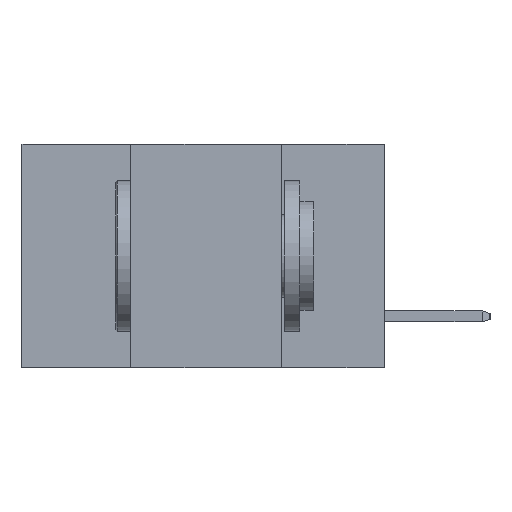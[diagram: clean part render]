
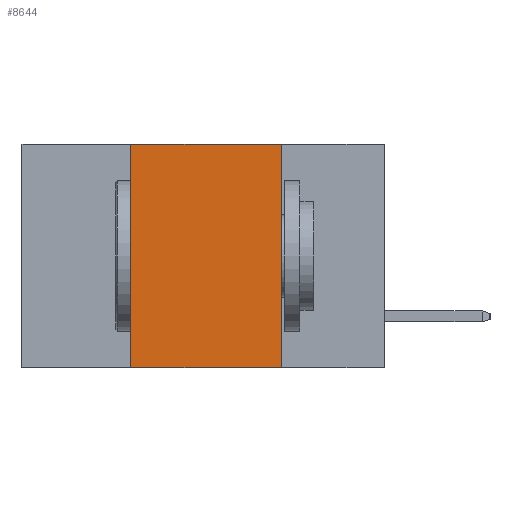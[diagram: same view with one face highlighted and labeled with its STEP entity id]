
A CAD part, left-side view. The second image highlights one B-rep face of the part: STEP entity #8644.
In plain terms, the highlighted planar face has unit normal (-1, 0, 0).
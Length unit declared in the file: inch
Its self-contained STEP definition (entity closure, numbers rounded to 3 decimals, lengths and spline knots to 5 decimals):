
#304 = LINE ( 'NONE', #5395, #17851 ) ;
#500 = DIRECTION ( 'NONE',  ( 1., 0., 0. ) ) ;
#922 = ORIENTED_EDGE ( 'NONE', *, *, #5301, .F. ) ;
#1385 = VECTOR ( 'NONE', #2786, 39.37008 ) ;
#1415 = ORIENTED_EDGE ( 'NONE', *, *, #14925, .F. ) ;
#1809 = CARTESIAN_POINT ( 'NONE',  ( 0., 0.17, 0. ) ) ;
#2786 = DIRECTION ( 'NONE',  ( 0., -1., 0. ) ) ;
#2829 = VECTOR ( 'NONE', #4533, 39.37008 ) ;
#3095 = CARTESIAN_POINT ( 'NONE',  ( 0., 0.6, -0.37 ) ) ;
#3645 = FACE_OUTER_BOUND ( 'NONE', #14759, .T. ) ;
#3710 = CARTESIAN_POINT ( 'NONE',  ( 0., 0.42, 0. ) ) ;
#3928 = CARTESIAN_POINT ( 'NONE',  ( 0., 0.42, -0.37 ) ) ;
#4533 = DIRECTION ( 'NONE',  ( 0., -1., 0. ) ) ;
#4705 = VECTOR ( 'NONE', #14823, 39.37008 ) ;
#5096 = AXIS2_PLACEMENT_3D ( 'NONE', #15878, #500, #10499 ) ;
#5301 = EDGE_CURVE ( 'NONE', #14714, #15538, #304, .T. ) ;
#5395 = CARTESIAN_POINT ( 'NONE',  ( 0., 0.17, 0. ) ) ;
#5481 = CARTESIAN_POINT ( 'NONE',  ( 0., 0.42, 0. ) ) ;
#5553 = DIRECTION ( 'NONE',  ( 0., 0., -1. ) ) ;
#8644 = ADVANCED_FACE ( 'NONE', ( #3645 ), #17155, .F. ) ;
#9843 = CARTESIAN_POINT ( 'NONE',  ( 0., 0.6, 0. ) ) ;
#10359 = LINE ( 'NONE', #3095, #2829 ) ;
#10499 = DIRECTION ( 'NONE',  ( 0., 0., -1. ) ) ;
#12109 = CARTESIAN_POINT ( 'NONE',  ( 0., 0.17, -0.37 ) ) ;
#12234 = EDGE_CURVE ( 'NONE', #13834, #15538, #10359, .T. ) ;
#12274 = ORIENTED_EDGE ( 'NONE', *, *, #13397, .F. ) ;
#13397 = EDGE_CURVE ( 'NONE', #17608, #14714, #15375, .T. ) ;
#13834 = VERTEX_POINT ( 'NONE', #3928 ) ;
#14714 = VERTEX_POINT ( 'NONE', #1809 ) ;
#14759 = EDGE_LOOP ( 'NONE', ( #922, #12274, #1415, #16617 ) ) ;
#14823 = DIRECTION ( 'NONE',  ( 0., 0., 1. ) ) ;
#14925 = EDGE_CURVE ( 'NONE', #13834, #17608, #15727, .T. ) ;
#15375 = LINE ( 'NONE', #9843, #1385 ) ;
#15538 = VERTEX_POINT ( 'NONE', #12109 ) ;
#15727 = LINE ( 'NONE', #3710, #4705 ) ;
#15878 = CARTESIAN_POINT ( 'NONE',  ( 0., 0.6, 0. ) ) ;
#16617 = ORIENTED_EDGE ( 'NONE', *, *, #12234, .T. ) ;
#17155 = PLANE ( 'NONE',  #5096 ) ;
#17608 = VERTEX_POINT ( 'NONE', #5481 ) ;
#17851 = VECTOR ( 'NONE', #5553, 39.37008 ) ;
